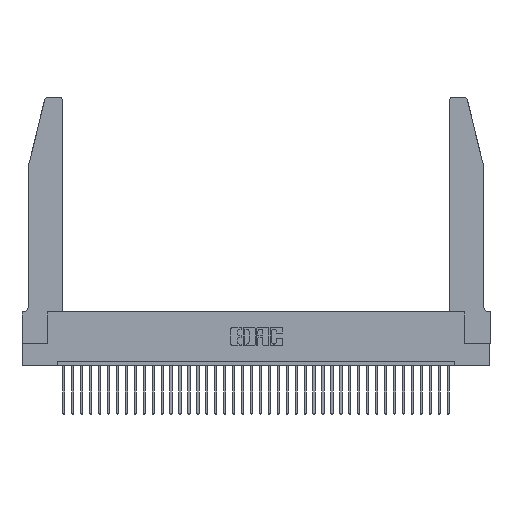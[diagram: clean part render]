
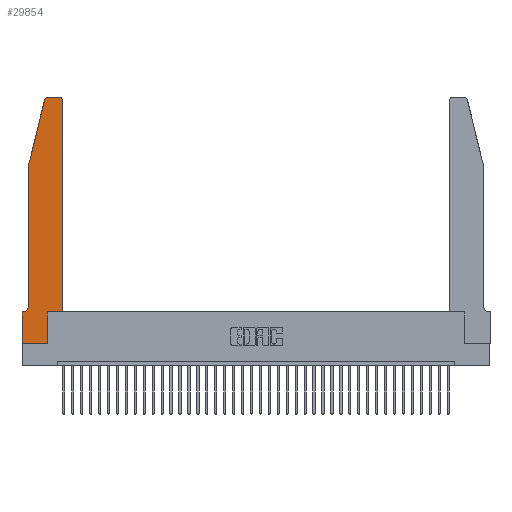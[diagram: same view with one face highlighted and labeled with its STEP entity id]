
A CAD part, top view. The second image highlights one B-rep face of the part: STEP entity #29854.
In plain terms, the highlighted planar face has unit normal (0, 0, 1).
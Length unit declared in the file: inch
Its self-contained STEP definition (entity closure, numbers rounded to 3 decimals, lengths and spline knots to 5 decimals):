
#591 = CARTESIAN_POINT ( 'NONE',  ( 0., 0., 0.37 ) ) ;
#824 = CARTESIAN_POINT ( 'NONE',  ( 0.2865, 0.35, 0.37 ) ) ;
#868 = VERTEX_POINT ( 'NONE', #29416 ) ;
#954 = ORIENTED_EDGE ( 'NONE', *, *, #11935, .T. ) ;
#1087 = VECTOR ( 'NONE', #20291, 39.37008 ) ;
#1509 = VERTEX_POINT ( 'NONE', #15002 ) ;
#1919 = VERTEX_POINT ( 'NONE', #36758 ) ;
#2573 = CARTESIAN_POINT ( 'NONE',  ( 0.0055, 0.42, 0.37 ) ) ;
#2664 = EDGE_CURVE ( 'NONE', #1509, #30559, #28162, .T. ) ;
#2860 = DIRECTION ( 'NONE',  ( 1., 0., 0. ) ) ;
#3427 = LINE ( 'NONE', #16475, #11593 ) ;
#3726 = DIRECTION ( 'NONE',  ( 0., 1., 0. ) ) ;
#4383 = EDGE_CURVE ( 'NONE', #30749, #31007, #27090, .T. ) ;
#4869 = EDGE_CURVE ( 'NONE', #11167, #868, #8016, .T. ) ;
#5337 = ORIENTED_EDGE ( 'NONE', *, *, #23941, .T. ) ;
#5447 = CARTESIAN_POINT ( 'NONE',  ( 0.25487, 2.72718, 0.37 ) ) ;
#6037 = ORIENTED_EDGE ( 'NONE', *, *, #34533, .T. ) ;
#6651 = VERTEX_POINT ( 'NONE', #5447 ) ;
#6934 = CARTESIAN_POINT ( 'NONE',  ( 0.4505, 0.35, 0.37 ) ) ;
#7191 = AXIS2_PLACEMENT_3D ( 'NONE', #14030, #14275, #16806 ) ;
#7551 = CIRCLE ( 'NONE', #36903, 0.03 ) ;
#7939 = DIRECTION ( 'NONE',  ( -0.239, -0.971, 0. ) ) ;
#8016 = LINE ( 'NONE', #16966, #14362 ) ;
#8987 = ORIENTED_EDGE ( 'NONE', *, *, #4383, .T. ) ;
#9295 = LINE ( 'NONE', #22421, #24745 ) ;
#9416 = CARTESIAN_POINT ( 'NONE',  ( 0.0755, 0.35, 0.37 ) ) ;
#10376 = CARTESIAN_POINT ( 'NONE',  ( 0., 0., 0.37 ) ) ;
#10722 = ORIENTED_EDGE ( 'NONE', *, *, #2664, .T. ) ;
#10937 = VECTOR ( 'NONE', #3726, 39.37008 ) ;
#11167 = VERTEX_POINT ( 'NONE', #16217 ) ;
#11242 = VECTOR ( 'NONE', #15532, 39.37008 ) ;
#11306 = CIRCLE ( 'NONE', #7191, 0.03 ) ;
#11548 = DIRECTION ( 'NONE',  ( -1., 0., 0. ) ) ;
#11593 = VECTOR ( 'NONE', #34183, 39.37008 ) ;
#11601 = ORIENTED_EDGE ( 'NONE', *, *, #22594, .T. ) ;
#11935 = EDGE_CURVE ( 'NONE', #30559, #33709, #17508, .T. ) ;
#11942 = LINE ( 'NONE', #32405, #1087 ) ;
#12765 = DIRECTION ( 'NONE',  ( 0., 0., 1. ) ) ;
#12985 = CARTESIAN_POINT ( 'NONE',  ( 0.2865, 0.35, 0.37 ) ) ;
#14030 = CARTESIAN_POINT ( 'NONE',  ( 0.4205, 2.72, 0.37 ) ) ;
#14275 = DIRECTION ( 'NONE',  ( 0., 0., 1. ) ) ;
#14362 = VECTOR ( 'NONE', #25200, 39.37008 ) ;
#14540 = LINE ( 'NONE', #18423, #22701 ) ;
#14793 = VECTOR ( 'NONE', #2860, 39.37008 ) ;
#15002 = CARTESIAN_POINT ( 'NONE',  ( 0.2865, 0., 0.37 ) ) ;
#15272 = DIRECTION ( 'NONE',  ( 0., -1., 0. ) ) ;
#15532 = DIRECTION ( 'NONE',  ( -1., 0., 0. ) ) ;
#15884 = DIRECTION ( 'NONE',  ( 0., 1., 0. ) ) ;
#16217 = CARTESIAN_POINT ( 'NONE',  ( 0.4205, 2.75, 0.37 ) ) ;
#16475 = CARTESIAN_POINT ( 'NONE',  ( 0.0755, 2., 0.37 ) ) ;
#16806 = DIRECTION ( 'NONE',  ( 1., 0., 0. ) ) ;
#16966 = CARTESIAN_POINT ( 'NONE',  ( 0.2605, 2.75, 0.37 ) ) ;
#17508 = LINE ( 'NONE', #23394, #14793 ) ;
#18423 = CARTESIAN_POINT ( 'NONE',  ( 0.4505, 0.35, 0.37 ) ) ;
#18852 = CARTESIAN_POINT ( 'NONE',  ( 0., 0.35, 0.37 ) ) ;
#19594 = VECTOR ( 'NONE', #15272, 39.37008 ) ;
#20035 = ORIENTED_EDGE ( 'NONE', *, *, #27978, .T. ) ;
#20251 = CARTESIAN_POINT ( 'NONE',  ( 0.4505, 2.72, 0.37 ) ) ;
#20291 = DIRECTION ( 'NONE',  ( 1., 0., 0. ) ) ;
#20320 = VERTEX_POINT ( 'NONE', #20251 ) ;
#22421 = CARTESIAN_POINT ( 'NONE',  ( 0.0755, 2., 0.37 ) ) ;
#22594 = EDGE_CURVE ( 'NONE', #20320, #11167, #11306, .T. ) ;
#22701 = VECTOR ( 'NONE', #15884, 39.37008 ) ;
#23346 = CARTESIAN_POINT ( 'NONE',  ( 0.284, 2.72, 0.37 ) ) ;
#23394 = CARTESIAN_POINT ( 'NONE',  ( 0.4505, 0.35, 0.37 ) ) ;
#23532 = ORIENTED_EDGE ( 'NONE', *, *, #34689, .T. ) ;
#23604 = CARTESIAN_POINT ( 'NONE',  ( 0., 0.35, 0.37 ) ) ;
#23832 = DIRECTION ( 'NONE',  ( 0., 0., 1. ) ) ;
#23843 = ORIENTED_EDGE ( 'NONE', *, *, #35532, .T. ) ;
#23941 = EDGE_CURVE ( 'NONE', #868, #6651, #7551, .T. ) ;
#24444 = AXIS2_PLACEMENT_3D ( 'NONE', #2573, #28790, #11548 ) ;
#24745 = VECTOR ( 'NONE', #7939, 39.37008 ) ;
#24982 = ORIENTED_EDGE ( 'NONE', *, *, #37064, .T. ) ;
#25200 = DIRECTION ( 'NONE',  ( -1., 0., 0. ) ) ;
#25968 = LINE ( 'NONE', #591, #19594 ) ;
#26619 = DIRECTION ( 'NONE',  ( 1., 0., 0. ) ) ;
#27090 = LINE ( 'NONE', #9416, #11242 ) ;
#27103 = PLANE ( 'NONE',  #29200 ) ;
#27206 = EDGE_LOOP ( 'NONE', ( #35463, #5337, #27737, #6037, #23532, #8987, #20035, #23843, #10722, #954, #24982, #11601 ) ) ;
#27737 = ORIENTED_EDGE ( 'NONE', *, *, #33258, .T. ) ;
#27978 = EDGE_CURVE ( 'NONE', #31007, #29969, #25968, .T. ) ;
#28162 = LINE ( 'NONE', #824, #10937 ) ;
#28790 = DIRECTION ( 'NONE',  ( 0., 0., -1. ) ) ;
#29200 = AXIS2_PLACEMENT_3D ( 'NONE', #18852, #12765, #33136 ) ;
#29416 = CARTESIAN_POINT ( 'NONE',  ( 0.284, 2.75, 0.37 ) ) ;
#29854 = ADVANCED_FACE ( 'NONE', ( #33612 ), #27103, .T. ) ;
#29969 = VERTEX_POINT ( 'NONE', #10376 ) ;
#30559 = VERTEX_POINT ( 'NONE', #12985 ) ;
#30749 = VERTEX_POINT ( 'NONE', #37391 ) ;
#31007 = VERTEX_POINT ( 'NONE', #23604 ) ;
#32030 = CIRCLE ( 'NONE', #24444, 0.07 ) ;
#32405 = CARTESIAN_POINT ( 'NONE',  ( 0., 0., 0.37 ) ) ;
#33136 = DIRECTION ( 'NONE',  ( 1., 0., 0. ) ) ;
#33258 = EDGE_CURVE ( 'NONE', #6651, #35071, #9295, .T. ) ;
#33534 = CARTESIAN_POINT ( 'NONE',  ( 0.0755, 2., 0.37 ) ) ;
#33612 = FACE_OUTER_BOUND ( 'NONE', #27206, .T. ) ;
#33709 = VERTEX_POINT ( 'NONE', #6934 ) ;
#34183 = DIRECTION ( 'NONE',  ( 0., -1., 0. ) ) ;
#34533 = EDGE_CURVE ( 'NONE', #35071, #1919, #3427, .T. ) ;
#34689 = EDGE_CURVE ( 'NONE', #1919, #30749, #32030, .T. ) ;
#35071 = VERTEX_POINT ( 'NONE', #33534 ) ;
#35463 = ORIENTED_EDGE ( 'NONE', *, *, #4869, .T. ) ;
#35532 = EDGE_CURVE ( 'NONE', #29969, #1509, #11942, .T. ) ;
#36758 = CARTESIAN_POINT ( 'NONE',  ( 0.0755, 0.42, 0.37 ) ) ;
#36903 = AXIS2_PLACEMENT_3D ( 'NONE', #23346, #23832, #26619 ) ;
#37064 = EDGE_CURVE ( 'NONE', #33709, #20320, #14540, .T. ) ;
#37391 = CARTESIAN_POINT ( 'NONE',  ( 0.0055, 0.35, 0.37 ) ) ;
